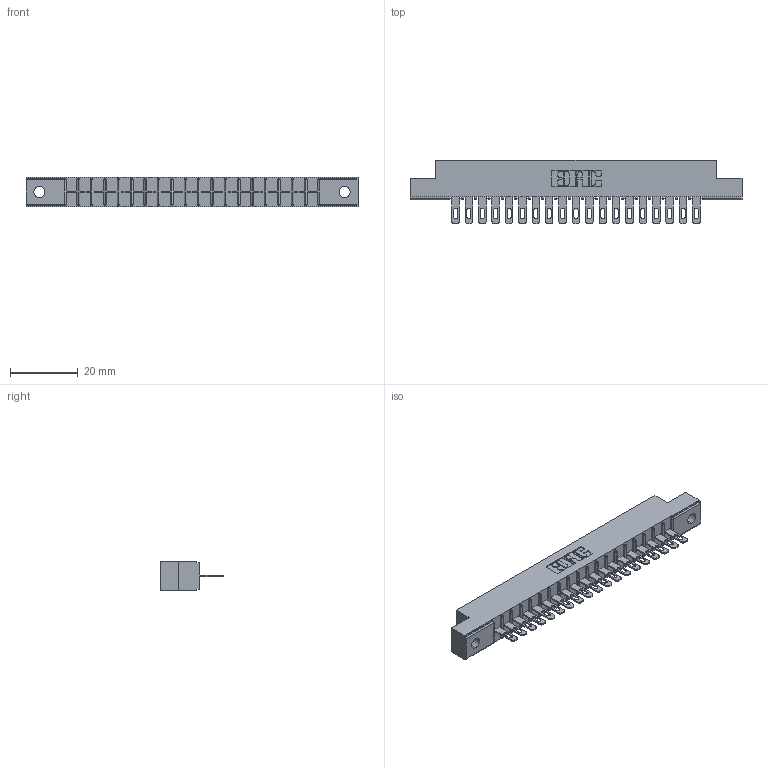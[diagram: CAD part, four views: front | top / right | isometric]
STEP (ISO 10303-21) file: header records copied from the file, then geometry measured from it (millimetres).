
FILE_DESCRIPTION (( 'STEP AP203' ), '1' );
FILE_NAME ('316-019-400-102.STEP', '2020-09-22T18:54:56', ( '' ), ( '' ), 'SwSTEP 2.0', 'SolidWorks 2020', '' );
FILE_SCHEMA (( 'CONFIG_CONTROL_DESIGN' ));
Length unit declared in the file: inch
Products named in the file (3): 306 Part_.128 Dia; 306-290-001_100; 316-019-400-102
Assembly tree (20 placements, depth 2):
  316-019-400-102
    306 Part_.128 Dia
    306-290-001_100  x19
Bounding box: 98.3 x 18.87 x 8.71 mm (x, y, z)
Volume: 6738 mm3; surface area: 9899.3 mm2
Topology: 20 solids, 20 shells, 1560 faces, 4401 edges, 2830 vertices
Faces by surface type: plane 1018, cylinder 466, sphere 76
Entity records: 20864 total; most frequent: CARTESIAN_POINT 3500, ORIENTED_EDGE 3466, DIRECTION 3455, EDGE_CURVE 1733, LINE 1341, VECTOR 1341, VERTEX_POINT 1102, AXIS2_PLACEMENT_3D 1057
